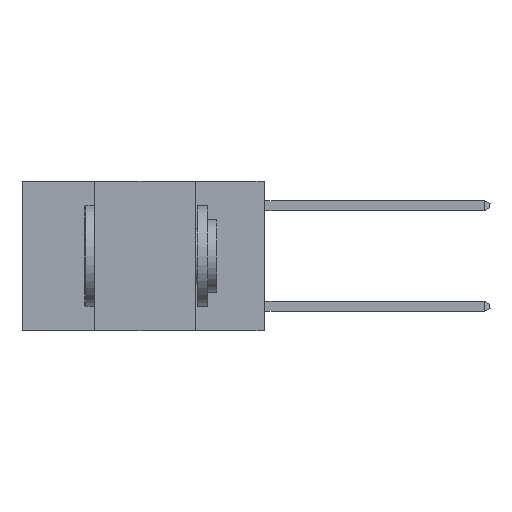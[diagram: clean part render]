
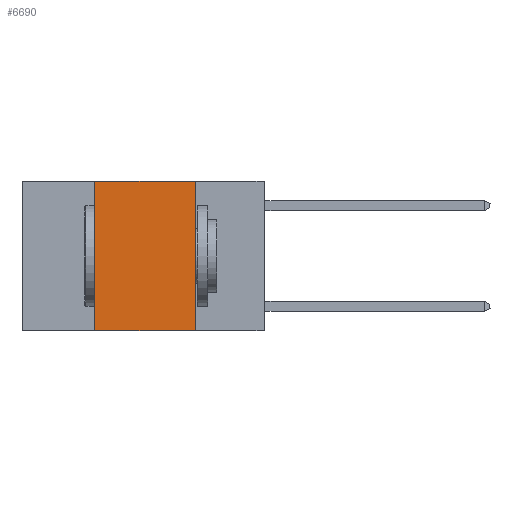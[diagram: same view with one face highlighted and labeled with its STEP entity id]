
A CAD part, left-side view. The second image highlights one B-rep face of the part: STEP entity #6690.
In plain terms, the highlighted planar face has unit normal (-1, 0, 0).
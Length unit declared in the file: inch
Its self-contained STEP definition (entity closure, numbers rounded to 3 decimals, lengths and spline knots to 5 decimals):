
#481 = CARTESIAN_POINT ( 'NONE',  ( 0., 0.6, -0.37 ) ) ;
#686 = AXIS2_PLACEMENT_3D ( 'NONE', #11971, #5451, #24202 ) ;
#1216 = DIRECTION ( 'NONE',  ( 0., 0., -1. ) ) ;
#1225 = ORIENTED_EDGE ( 'NONE', *, *, #13399, .F. ) ;
#2778 = LINE ( 'NONE', #17356, #21252 ) ;
#3498 = ORIENTED_EDGE ( 'NONE', *, *, #8409, .T. ) ;
#4395 = VERTEX_POINT ( 'NONE', #17134 ) ;
#4916 = CARTESIAN_POINT ( 'NONE',  ( 0., 0.42, 0. ) ) ;
#5309 = VERTEX_POINT ( 'NONE', #4916 ) ;
#5451 = DIRECTION ( 'NONE',  ( 1., 0., 0. ) ) ;
#6690 = ADVANCED_FACE ( 'NONE', ( #20319 ), #13713, .F. ) ;
#7981 = VECTOR ( 'NONE', #20275, 39.37008 ) ;
#8386 = VERTEX_POINT ( 'NONE', #21258 ) ;
#8409 = EDGE_CURVE ( 'NONE', #4395, #8386, #18993, .T. ) ;
#9204 = ORIENTED_EDGE ( 'NONE', *, *, #11316, .F. ) ;
#9854 = CARTESIAN_POINT ( 'NONE',  ( 0., 0.17, 0. ) ) ;
#10132 = CARTESIAN_POINT ( 'NONE',  ( 0., 0.42, 0. ) ) ;
#11316 = EDGE_CURVE ( 'NONE', #13763, #8386, #19992, .T. ) ;
#11971 = CARTESIAN_POINT ( 'NONE',  ( 0., 0.6, 0. ) ) ;
#12913 = DIRECTION ( 'NONE',  ( 0., -1., 0. ) ) ;
#13177 = DIRECTION ( 'NONE',  ( 0., -1., 0. ) ) ;
#13399 = EDGE_CURVE ( 'NONE', #5309, #13763, #2778, .T. ) ;
#13713 = PLANE ( 'NONE',  #686 ) ;
#13763 = VERTEX_POINT ( 'NONE', #16804 ) ;
#15711 = VECTOR ( 'NONE', #13177, 39.37008 ) ;
#16109 = LINE ( 'NONE', #10132, #7981 ) ;
#16804 = CARTESIAN_POINT ( 'NONE',  ( 0., 0.17, 0. ) ) ;
#17134 = CARTESIAN_POINT ( 'NONE',  ( 0., 0.42, -0.37 ) ) ;
#17288 = EDGE_CURVE ( 'NONE', #4395, #5309, #16109, .T. ) ;
#17356 = CARTESIAN_POINT ( 'NONE',  ( 0., 0.6, 0. ) ) ;
#18993 = LINE ( 'NONE', #481, #15711 ) ;
#19503 = VECTOR ( 'NONE', #1216, 39.37008 ) ;
#19992 = LINE ( 'NONE', #9854, #19503 ) ;
#20275 = DIRECTION ( 'NONE',  ( 0., 0., 1. ) ) ;
#20319 = FACE_OUTER_BOUND ( 'NONE', #24232, .T. ) ;
#21252 = VECTOR ( 'NONE', #12913, 39.37008 ) ;
#21258 = CARTESIAN_POINT ( 'NONE',  ( 0., 0.17, -0.37 ) ) ;
#22727 = ORIENTED_EDGE ( 'NONE', *, *, #17288, .F. ) ;
#24202 = DIRECTION ( 'NONE',  ( 0., 0., -1. ) ) ;
#24232 = EDGE_LOOP ( 'NONE', ( #9204, #1225, #22727, #3498 ) ) ;
